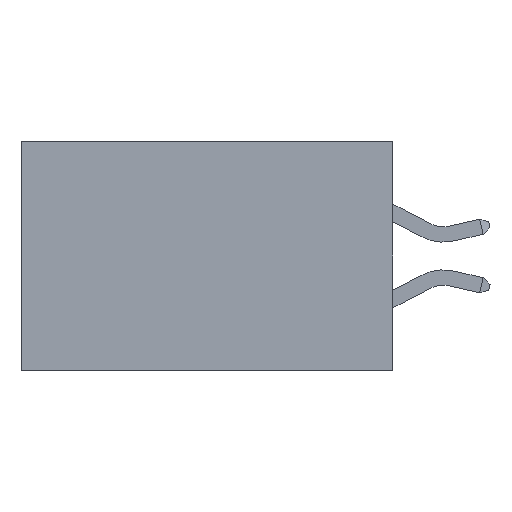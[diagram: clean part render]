
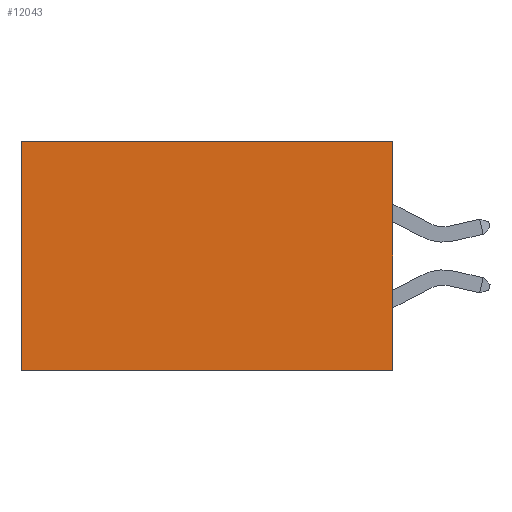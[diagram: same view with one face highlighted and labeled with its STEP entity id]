
A CAD part, left-side view. The second image highlights one B-rep face of the part: STEP entity #12043.
In plain terms, the highlighted planar face has unit normal (-1, 0, 0).
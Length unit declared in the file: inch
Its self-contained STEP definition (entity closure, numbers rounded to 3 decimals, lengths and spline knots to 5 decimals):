
#237 = VERTEX_POINT ( 'NONE', #28795 ) ;
#936 = EDGE_CURVE ( 'NONE', #17732, #8715, #20789, .T. ) ;
#4844 = VECTOR ( 'NONE', #18033, 39.37008 ) ;
#6922 = DIRECTION ( 'NONE',  ( 0., 0., -1. ) ) ;
#7038 = CARTESIAN_POINT ( 'NONE',  ( 0.2875, 0., 0. ) ) ;
#8715 = VERTEX_POINT ( 'NONE', #25315 ) ;
#11408 = ORIENTED_EDGE ( 'NONE', *, *, #19754, .T. ) ;
#12022 = DIRECTION ( 'NONE',  ( 0., 0., -1. ) ) ;
#12043 = ADVANCED_FACE ( 'NONE', ( #24036 ), #29282, .F. ) ;
#13153 = LINE ( 'NONE', #29104, #19654 ) ;
#14419 = LINE ( 'NONE', #36165, #31943 ) ;
#17732 = VERTEX_POINT ( 'NONE', #27611 ) ;
#18033 = DIRECTION ( 'NONE',  ( 0., 1., 0. ) ) ;
#19280 = EDGE_CURVE ( 'NONE', #25273, #237, #13153, .T. ) ;
#19654 = VECTOR ( 'NONE', #28725, 39.37008 ) ;
#19754 = EDGE_CURVE ( 'NONE', #17732, #25273, #14419, .T. ) ;
#20347 = VECTOR ( 'NONE', #12022, 39.37008 ) ;
#20789 = LINE ( 'NONE', #28749, #20347 ) ;
#24036 = FACE_OUTER_BOUND ( 'NONE', #27395, .T. ) ;
#24837 = ORIENTED_EDGE ( 'NONE', *, *, #30509, .F. ) ;
#25148 = DIRECTION ( 'NONE',  ( 0., 1., 0. ) ) ;
#25273 = VERTEX_POINT ( 'NONE', #26752 ) ;
#25315 = CARTESIAN_POINT ( 'NONE',  ( 0.2875, 0., -0.37 ) ) ;
#26752 = CARTESIAN_POINT ( 'NONE',  ( 0.2875, 0.6, 0. ) ) ;
#27395 = EDGE_LOOP ( 'NONE', ( #28999, #24837, #30965, #11408 ) ) ;
#27611 = CARTESIAN_POINT ( 'NONE',  ( 0.2875, 0., 0. ) ) ;
#28009 = LINE ( 'NONE', #29284, #4844 ) ;
#28725 = DIRECTION ( 'NONE',  ( 0., 0., -1. ) ) ;
#28749 = CARTESIAN_POINT ( 'NONE',  ( 0.2875, 0., 0. ) ) ;
#28795 = CARTESIAN_POINT ( 'NONE',  ( 0.2875, 0.6, -0.37 ) ) ;
#28999 = ORIENTED_EDGE ( 'NONE', *, *, #19280, .T. ) ;
#29104 = CARTESIAN_POINT ( 'NONE',  ( 0.2875, 0.6, 0. ) ) ;
#29282 = PLANE ( 'NONE',  #35568 ) ;
#29284 = CARTESIAN_POINT ( 'NONE',  ( 0.2875, 0., -0.37 ) ) ;
#30509 = EDGE_CURVE ( 'NONE', #8715, #237, #28009, .T. ) ;
#30965 = ORIENTED_EDGE ( 'NONE', *, *, #936, .F. ) ;
#31943 = VECTOR ( 'NONE', #25148, 39.37008 ) ;
#32229 = DIRECTION ( 'NONE',  ( 1., 0., 0. ) ) ;
#35568 = AXIS2_PLACEMENT_3D ( 'NONE', #7038, #32229, #6922 ) ;
#36165 = CARTESIAN_POINT ( 'NONE',  ( 0.2875, 0., 0. ) ) ;
